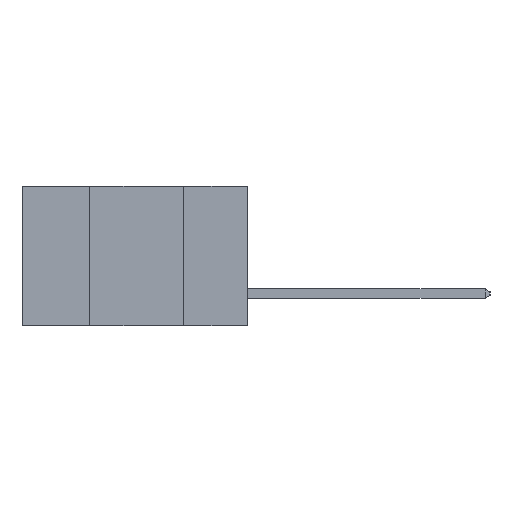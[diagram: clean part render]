
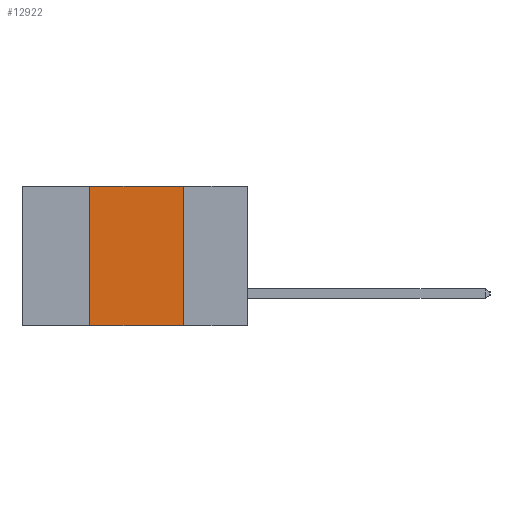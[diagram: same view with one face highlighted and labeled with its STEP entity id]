
A CAD part, left-side view. The second image highlights one B-rep face of the part: STEP entity #12922.
In plain terms, the highlighted planar face has unit normal (-1, 0, 0).
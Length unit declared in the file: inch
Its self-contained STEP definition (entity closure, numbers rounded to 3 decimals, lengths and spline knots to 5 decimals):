
#26 = VECTOR ( 'NONE', #9784, 39.37008 ) ;
#65 = VERTEX_POINT ( 'NONE', #14643 ) ;
#286 = VERTEX_POINT ( 'NONE', #15333 ) ;
#1460 = ORIENTED_EDGE ( 'NONE', *, *, #5995, .T. ) ;
#1545 = CARTESIAN_POINT ( 'NONE',  ( 0., 0.6, 0. ) ) ;
#1757 = VERTEX_POINT ( 'NONE', #5831 ) ;
#2243 = CARTESIAN_POINT ( 'NONE',  ( 0., 0.17, 0. ) ) ;
#4450 = LINE ( 'NONE', #4550, #7282 ) ;
#4550 = CARTESIAN_POINT ( 'NONE',  ( 0., 0.6, -0.37 ) ) ;
#4710 = EDGE_LOOP ( 'NONE', ( #7616, #14979, #10881, #1460 ) ) ;
#5831 = CARTESIAN_POINT ( 'NONE',  ( 0., 0.17, -0.37 ) ) ;
#5995 = EDGE_CURVE ( 'NONE', #65, #1757, #4450, .T. ) ;
#6018 = LINE ( 'NONE', #13290, #26 ) ;
#6428 = EDGE_CURVE ( 'NONE', #13680, #286, #7652, .T. ) ;
#6586 = PLANE ( 'NONE',  #10483 ) ;
#7282 = VECTOR ( 'NONE', #12864, 39.37008 ) ;
#7616 = ORIENTED_EDGE ( 'NONE', *, *, #9238, .F. ) ;
#7652 = LINE ( 'NONE', #12495, #10435 ) ;
#7804 = DIRECTION ( 'NONE',  ( 0., 0., -1. ) ) ;
#8426 = EDGE_CURVE ( 'NONE', #65, #13680, #6018, .T. ) ;
#9238 = EDGE_CURVE ( 'NONE', #286, #1757, #12665, .T. ) ;
#9784 = DIRECTION ( 'NONE',  ( 0., 0., 1. ) ) ;
#9946 = VECTOR ( 'NONE', #10603, 39.37008 ) ;
#10435 = VECTOR ( 'NONE', #12184, 39.37008 ) ;
#10483 = AXIS2_PLACEMENT_3D ( 'NONE', #1545, #14818, #7804 ) ;
#10603 = DIRECTION ( 'NONE',  ( 0., 0., -1. ) ) ;
#10881 = ORIENTED_EDGE ( 'NONE', *, *, #8426, .F. ) ;
#12184 = DIRECTION ( 'NONE',  ( 0., -1., 0. ) ) ;
#12495 = CARTESIAN_POINT ( 'NONE',  ( 0., 0.6, 0. ) ) ;
#12665 = LINE ( 'NONE', #2243, #9946 ) ;
#12864 = DIRECTION ( 'NONE',  ( 0., -1., 0. ) ) ;
#12922 = ADVANCED_FACE ( 'NONE', ( #13943 ), #6586, .F. ) ;
#13290 = CARTESIAN_POINT ( 'NONE',  ( 0., 0.42, 0. ) ) ;
#13680 = VERTEX_POINT ( 'NONE', #14878 ) ;
#13943 = FACE_OUTER_BOUND ( 'NONE', #4710, .T. ) ;
#14643 = CARTESIAN_POINT ( 'NONE',  ( 0., 0.42, -0.37 ) ) ;
#14818 = DIRECTION ( 'NONE',  ( 1., 0., 0. ) ) ;
#14878 = CARTESIAN_POINT ( 'NONE',  ( 0., 0.42, 0. ) ) ;
#14979 = ORIENTED_EDGE ( 'NONE', *, *, #6428, .F. ) ;
#15333 = CARTESIAN_POINT ( 'NONE',  ( 0., 0.17, 0. ) ) ;
